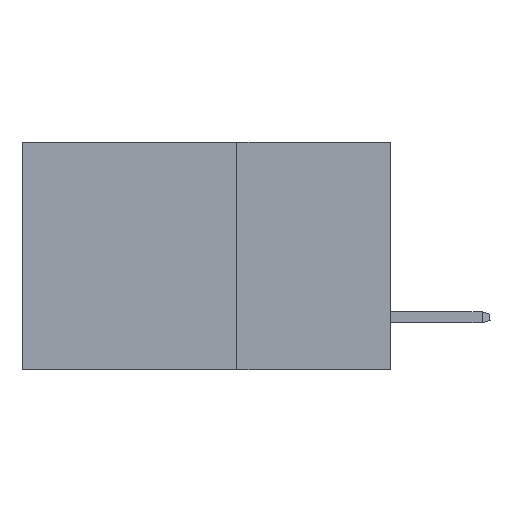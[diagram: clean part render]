
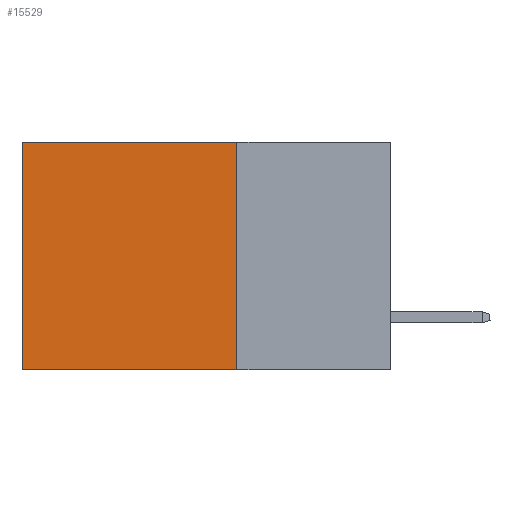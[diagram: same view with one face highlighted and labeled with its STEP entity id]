
A CAD part, left-side view. The second image highlights one B-rep face of the part: STEP entity #15529.
In plain terms, the highlighted planar face has unit normal (-1, 0, 0).
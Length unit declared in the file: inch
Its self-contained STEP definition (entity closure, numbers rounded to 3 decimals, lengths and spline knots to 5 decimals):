
#718 = VECTOR ( 'NONE', #5481, 39.37008 ) ;
#1198 = EDGE_CURVE ( 'NONE', #3138, #11884, #39159, .T. ) ;
#2595 = ORIENTED_EDGE ( 'NONE', *, *, #23752, .T. ) ;
#3138 = VERTEX_POINT ( 'NONE', #27153 ) ;
#5481 = DIRECTION ( 'NONE',  ( 0., 0., -1. ) ) ;
#6160 = VECTOR ( 'NONE', #14848, 39.37008 ) ;
#11504 = CARTESIAN_POINT ( 'NONE',  ( 0.2875, 0.25, 0. ) ) ;
#11884 = VERTEX_POINT ( 'NONE', #26694 ) ;
#14287 = DIRECTION ( 'NONE',  ( 1., 0., 0. ) ) ;
#14848 = DIRECTION ( 'NONE',  ( 0., 1., 0. ) ) ;
#14927 = VERTEX_POINT ( 'NONE', #31305 ) ;
#15529 = ADVANCED_FACE ( 'NONE', ( #20138 ), #24222, .F. ) ;
#16221 = EDGE_CURVE ( 'NONE', #14927, #3138, #25384, .T. ) ;
#16728 = VERTEX_POINT ( 'NONE', #30454 ) ;
#17216 = ORIENTED_EDGE ( 'NONE', *, *, #1198, .F. ) ;
#17978 = DIRECTION ( 'NONE',  ( 0., 0., -1. ) ) ;
#18258 = LINE ( 'NONE', #38121, #718 ) ;
#19113 = LINE ( 'NONE', #34437, #6160 ) ;
#20138 = FACE_OUTER_BOUND ( 'NONE', #39736, .T. ) ;
#23016 = CARTESIAN_POINT ( 'NONE',  ( 0.2875, 0.25, -0.37 ) ) ;
#23752 = EDGE_CURVE ( 'NONE', #16728, #11884, #18258, .T. ) ;
#24222 = PLANE ( 'NONE',  #28152 ) ;
#25384 = LINE ( 'NONE', #11504, #31050 ) ;
#26167 = DIRECTION ( 'NONE',  ( 0., 1., 0. ) ) ;
#26694 = CARTESIAN_POINT ( 'NONE',  ( 0.2875, 0.6, -0.37 ) ) ;
#27153 = CARTESIAN_POINT ( 'NONE',  ( 0.2875, 0.25, -0.37 ) ) ;
#28152 = AXIS2_PLACEMENT_3D ( 'NONE', #34024, #14287, #40874 ) ;
#30454 = CARTESIAN_POINT ( 'NONE',  ( 0.2875, 0.6, 0. ) ) ;
#30815 = EDGE_CURVE ( 'NONE', #14927, #16728, #19113, .T. ) ;
#31050 = VECTOR ( 'NONE', #17978, 39.37008 ) ;
#31191 = ORIENTED_EDGE ( 'NONE', *, *, #30815, .T. ) ;
#31305 = CARTESIAN_POINT ( 'NONE',  ( 0.2875, 0.25, 0. ) ) ;
#31778 = ORIENTED_EDGE ( 'NONE', *, *, #16221, .F. ) ;
#34024 = CARTESIAN_POINT ( 'NONE',  ( 0.2875, 0.25, 0. ) ) ;
#34437 = CARTESIAN_POINT ( 'NONE',  ( 0.2875, 0.25, 0. ) ) ;
#38121 = CARTESIAN_POINT ( 'NONE',  ( 0.2875, 0.6, 0. ) ) ;
#39159 = LINE ( 'NONE', #23016, #42798 ) ;
#39736 = EDGE_LOOP ( 'NONE', ( #2595, #17216, #31778, #31191 ) ) ;
#40874 = DIRECTION ( 'NONE',  ( 0., 0., -1. ) ) ;
#42798 = VECTOR ( 'NONE', #26167, 39.37008 ) ;
